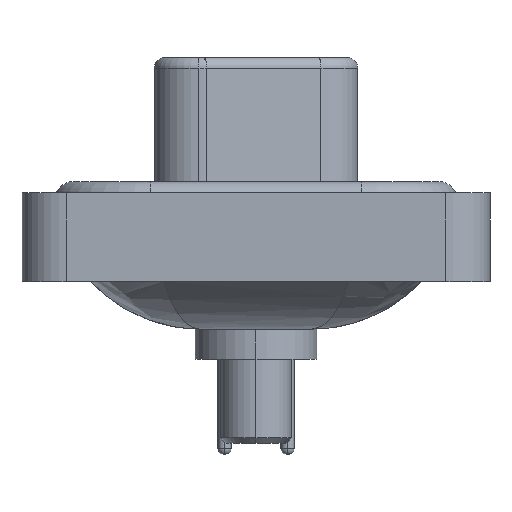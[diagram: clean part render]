
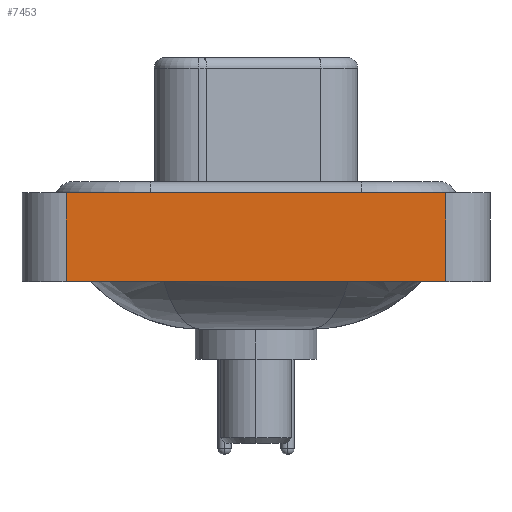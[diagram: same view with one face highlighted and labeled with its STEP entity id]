
A CAD part, left-side view. The second image highlights one B-rep face of the part: STEP entity #7453.
In plain terms, the highlighted planar face has unit normal (-1, 0, 0).
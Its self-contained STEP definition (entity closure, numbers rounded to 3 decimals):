
#1107 = DIRECTION ( 'NONE',  ( 0., 0., 1. ) ) ;
#1159 = AXIS2_PLACEMENT_3D ( 'NONE', #22581, #6668, #1107 ) ;
#1488 = VECTOR ( 'NONE', #22432, 1000. ) ;
#2141 = LINE ( 'NONE', #17818, #12037 ) ;
#2220 = ORIENTED_EDGE ( 'NONE', *, *, #11592, .T. ) ;
#2289 = EDGE_CURVE ( 'NONE', #17846, #13233, #2141, .T. ) ;
#2299 = ORIENTED_EDGE ( 'NONE', *, *, #2289, .T. ) ;
#2414 = CARTESIAN_POINT ( 'NONE',  ( -7.35, -8.55, 0.4 ) ) ;
#3296 = CARTESIAN_POINT ( 'NONE',  ( -7.35, 8.55, 0.4 ) ) ;
#3842 = ORIENTED_EDGE ( 'NONE', *, *, #20076, .F. ) ;
#4751 = CARTESIAN_POINT ( 'NONE',  ( -7.35, 8.55, -3.6 ) ) ;
#6043 = LINE ( 'NONE', #20093, #22606 ) ;
#6668 = DIRECTION ( 'NONE',  ( -1., 0., 0. ) ) ;
#7223 = VECTOR ( 'NONE', #22493, 1000. ) ;
#7453 = ADVANCED_FACE ( 'NONE', ( #18964 ), #9926, .T. ) ;
#8132 = CARTESIAN_POINT ( 'NONE',  ( -7.35, 8.55, -3.6 ) ) ;
#9926 = PLANE ( 'NONE',  #1159 ) ;
#10105 = CARTESIAN_POINT ( 'NONE',  ( -7.35, -8.55, -3.6 ) ) ;
#10359 = LINE ( 'NONE', #4751, #1488 ) ;
#11592 = EDGE_CURVE ( 'NONE', #17599, #17846, #6043, .T. ) ;
#12037 = VECTOR ( 'NONE', #14582, 1000. ) ;
#12722 = EDGE_LOOP ( 'NONE', ( #2299, #17673, #3842, #2220 ) ) ;
#13233 = VERTEX_POINT ( 'NONE', #2414 ) ;
#13947 = VERTEX_POINT ( 'NONE', #3296 ) ;
#14582 = DIRECTION ( 'NONE',  ( 0., 0., 1. ) ) ;
#15167 = CARTESIAN_POINT ( 'NONE',  ( -7.35, -8.55, 0.4 ) ) ;
#16615 = DIRECTION ( 'NONE',  ( 0., -1., 0. ) ) ;
#16901 = EDGE_CURVE ( 'NONE', #13947, #13233, #22380, .T. ) ;
#17599 = VERTEX_POINT ( 'NONE', #8132 ) ;
#17673 = ORIENTED_EDGE ( 'NONE', *, *, #16901, .F. ) ;
#17818 = CARTESIAN_POINT ( 'NONE',  ( -7.35, -8.55, -3.6 ) ) ;
#17846 = VERTEX_POINT ( 'NONE', #10105 ) ;
#18964 = FACE_OUTER_BOUND ( 'NONE', #12722, .T. ) ;
#20076 = EDGE_CURVE ( 'NONE', #17599, #13947, #10359, .T. ) ;
#20093 = CARTESIAN_POINT ( 'NONE',  ( -7.35, -8.55, -3.6 ) ) ;
#22380 = LINE ( 'NONE', #15167, #7223 ) ;
#22432 = DIRECTION ( 'NONE',  ( 0., 0., 1. ) ) ;
#22493 = DIRECTION ( 'NONE',  ( 0., -1., 0. ) ) ;
#22581 = CARTESIAN_POINT ( 'NONE',  ( -7.35, -8.55, -3.6 ) ) ;
#22606 = VECTOR ( 'NONE', #16615, 1000. ) ;
